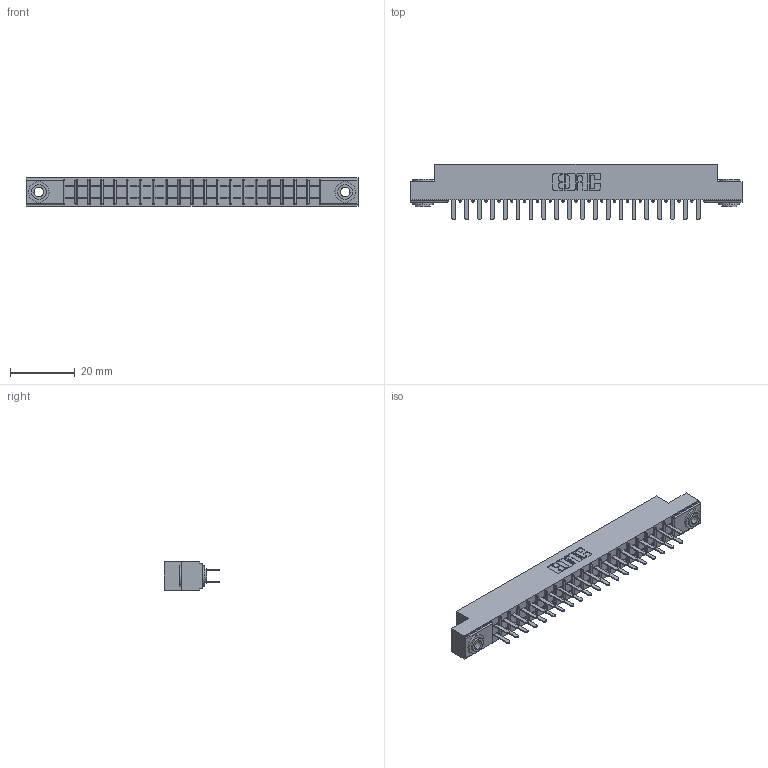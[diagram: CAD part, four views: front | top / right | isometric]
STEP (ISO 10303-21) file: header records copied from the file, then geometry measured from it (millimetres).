
FILE_DESCRIPTION (( 'STEP AP203' ), '1' );
FILE_NAME ('305-040-520-503.STEP', '2019-09-09T18:55:47', ( '' ), ( '' ), 'SwSTEP 2.0', 'SolidWorks 2016', '' );
FILE_SCHEMA (( 'CONFIG_CONTROL_DESIGN' ));
Length unit declared in the file: inch
Products named in the file (4): 305 Part_.156 Dia; 305-290-001_520; 345-250-002_345-250-002-102; 305-040-520-503
Assembly tree (43 placements, depth 2):
  305-040-520-503
    305 Part_.156 Dia
    305-290-001_520  x40
    345-250-002_345-250-002-102  x2
Bounding box: 102.26 x 17.09 x 8.71 mm (x, y, z)
Volume: 6133.8 mm3; surface area: 12370.3 mm2
Topology: 43 solids, 43 shells, 2008 faces, 5688 edges, 3680 vertices
Faces by surface type: plane 1172, cylinder 748, sphere 80, cone 8
Entity records: 25278 total; most frequent: CARTESIAN_POINT 4163, ORIENTED_EDGE 4120, DIRECTION 4060, EDGE_CURVE 2060, VECTOR 1634, LINE 1634, VERTEX_POINT 1316, AXIS2_PLACEMENT_3D 1213
